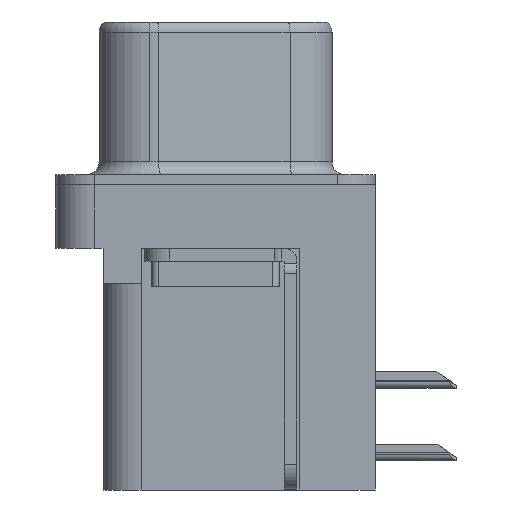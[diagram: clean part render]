
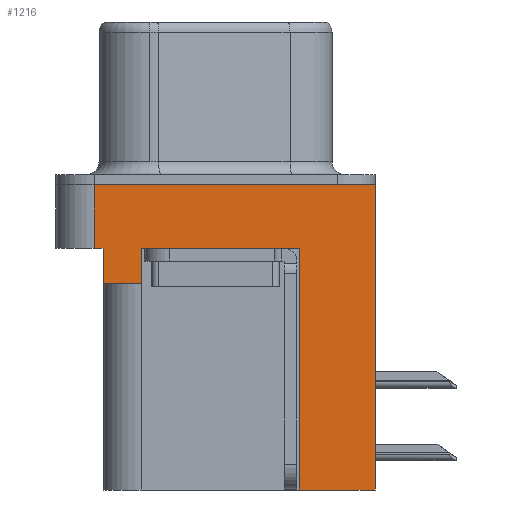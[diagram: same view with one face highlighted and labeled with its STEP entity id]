
A CAD part, left-side view. The second image highlights one B-rep face of the part: STEP entity #1216.
In plain terms, the highlighted planar face has unit normal (-1, 0, 0).
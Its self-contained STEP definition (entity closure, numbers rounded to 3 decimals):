
#251 = DIRECTION ( 'NONE',  ( 0., 0., 1. ) ) ;
#421 = EDGE_CURVE ( 'NONE', #2257, #21516, #5055, .T. ) ;
#840 = VECTOR ( 'NONE', #251, 1000. ) ;
#1216 = ADVANCED_FACE ( 'NONE', ( #18706 ), #11999, .T. ) ;
#1802 = DIRECTION ( 'NONE',  ( 0., 0., 1. ) ) ;
#2257 = VERTEX_POINT ( 'NONE', #19179 ) ;
#2380 = VERTEX_POINT ( 'NONE', #13673 ) ;
#2423 = EDGE_CURVE ( 'NONE', #16780, #21516, #10642, .T. ) ;
#2536 = CARTESIAN_POINT ( 'NONE',  ( -2.91, -6.275, 0. ) ) ;
#3403 = VERTEX_POINT ( 'NONE', #19864 ) ;
#3629 = VERTEX_POINT ( 'NONE', #9405 ) ;
#3684 = LINE ( 'NONE', #2536, #14914 ) ;
#3899 = VECTOR ( 'NONE', #12771, 1000. ) ;
#4153 = CARTESIAN_POINT ( 'NONE',  ( -2.91, 2.895, -3.9 ) ) ;
#4508 = VECTOR ( 'NONE', #14130, 1000. ) ;
#4547 = LINE ( 'NONE', #10882, #23035 ) ;
#4643 = AXIS2_PLACEMENT_3D ( 'NONE', #20243, #8157, #12079 ) ;
#5055 = LINE ( 'NONE', #24226, #22276 ) ;
#5524 = ORIENTED_EDGE ( 'NONE', *, *, #19649, .F. ) ;
#5547 = EDGE_CURVE ( 'NONE', #2380, #3403, #16661, .T. ) ;
#5751 = LINE ( 'NONE', #8375, #22029 ) ;
#6090 = LINE ( 'NONE', #26316, #4508 ) ;
#6662 = EDGE_CURVE ( 'NONE', #9541, #9669, #12764, .T. ) ;
#8157 = DIRECTION ( 'NONE',  ( -1., 0., 0. ) ) ;
#8258 = CARTESIAN_POINT ( 'NONE',  ( -2.91, 4.425, -3.9 ) ) ;
#8375 = CARTESIAN_POINT ( 'NONE',  ( -2.91, -3.295, -12. ) ) ;
#9310 = ORIENTED_EDGE ( 'NONE', *, *, #20270, .F. ) ;
#9405 = CARTESIAN_POINT ( 'NONE',  ( -2.91, 4.775, 0. ) ) ;
#9541 = VERTEX_POINT ( 'NONE', #11743 ) ;
#9669 = VERTEX_POINT ( 'NONE', #13704 ) ;
#9753 = DIRECTION ( 'NONE',  ( 0., 1., 0. ) ) ;
#10254 = LINE ( 'NONE', #24213, #19192 ) ;
#10642 = LINE ( 'NONE', #25937, #10959 ) ;
#10882 = CARTESIAN_POINT ( 'NONE',  ( -2.91, 4.775, -2.5 ) ) ;
#10896 = ORIENTED_EDGE ( 'NONE', *, *, #2423, .T. ) ;
#10959 = VECTOR ( 'NONE', #19844, 1000. ) ;
#11530 = CARTESIAN_POINT ( 'NONE',  ( -2.91, -6.275, -2.5 ) ) ;
#11743 = CARTESIAN_POINT ( 'NONE',  ( -2.91, 4.775, -2.5 ) ) ;
#11999 = PLANE ( 'NONE',  #4643 ) ;
#12079 = DIRECTION ( 'NONE',  ( 0., 0., 1. ) ) ;
#12124 = CARTESIAN_POINT ( 'NONE',  ( -2.91, 4.425, -3.9 ) ) ;
#12764 = LINE ( 'NONE', #11530, #18198 ) ;
#12771 = DIRECTION ( 'NONE',  ( 0., 0., 1. ) ) ;
#13673 = CARTESIAN_POINT ( 'NONE',  ( -2.91, -6.275, -12. ) ) ;
#13704 = CARTESIAN_POINT ( 'NONE',  ( -2.91, 4.425, -2.5 ) ) ;
#14130 = DIRECTION ( 'NONE',  ( 0., 0., 1. ) ) ;
#14210 = CARTESIAN_POINT ( 'NONE',  ( -2.91, -3.295, -2.5 ) ) ;
#14914 = VECTOR ( 'NONE', #24719, 1000. ) ;
#16099 = ORIENTED_EDGE ( 'NONE', *, *, #18065, .F. ) ;
#16661 = LINE ( 'NONE', #26484, #3899 ) ;
#16780 = VERTEX_POINT ( 'NONE', #18394 ) ;
#18065 = EDGE_CURVE ( 'NONE', #23569, #22270, #10254, .T. ) ;
#18198 = VECTOR ( 'NONE', #23469, 1000. ) ;
#18248 = EDGE_CURVE ( 'NONE', #2380, #2257, #5751, .T. ) ;
#18394 = CARTESIAN_POINT ( 'NONE',  ( -2.91, 2.895, -2.5 ) ) ;
#18706 = FACE_OUTER_BOUND ( 'NONE', #19726, .T. ) ;
#19179 = CARTESIAN_POINT ( 'NONE',  ( -2.91, -3.295, -12. ) ) ;
#19192 = VECTOR ( 'NONE', #9753, 1000. ) ;
#19393 = ORIENTED_EDGE ( 'NONE', *, *, #25135, .T. ) ;
#19649 = EDGE_CURVE ( 'NONE', #22270, #9669, #25145, .T. ) ;
#19726 = EDGE_LOOP ( 'NONE', ( #9310, #20275, #21149, #5524, #16099, #19393, #10896, #19888, #24588, #23963 ) ) ;
#19844 = DIRECTION ( 'NONE',  ( 0., -1., 0. ) ) ;
#19864 = CARTESIAN_POINT ( 'NONE',  ( -2.91, -6.275, 0. ) ) ;
#19888 = ORIENTED_EDGE ( 'NONE', *, *, #421, .F. ) ;
#20243 = CARTESIAN_POINT ( 'NONE',  ( -2.91, -6.275, -2.5 ) ) ;
#20270 = EDGE_CURVE ( 'NONE', #3629, #3403, #3684, .T. ) ;
#20275 = ORIENTED_EDGE ( 'NONE', *, *, #21636, .F. ) ;
#20986 = DIRECTION ( 'NONE',  ( 0., 1., 0. ) ) ;
#21095 = DIRECTION ( 'NONE',  ( 0., 0., 1. ) ) ;
#21149 = ORIENTED_EDGE ( 'NONE', *, *, #6662, .T. ) ;
#21516 = VERTEX_POINT ( 'NONE', #14210 ) ;
#21636 = EDGE_CURVE ( 'NONE', #9541, #3629, #4547, .T. ) ;
#22029 = VECTOR ( 'NONE', #20986, 1000. ) ;
#22270 = VERTEX_POINT ( 'NONE', #8258 ) ;
#22276 = VECTOR ( 'NONE', #1802, 1000. ) ;
#23035 = VECTOR ( 'NONE', #21095, 1000. ) ;
#23469 = DIRECTION ( 'NONE',  ( 0., -1., 0. ) ) ;
#23569 = VERTEX_POINT ( 'NONE', #4153 ) ;
#23963 = ORIENTED_EDGE ( 'NONE', *, *, #5547, .T. ) ;
#24213 = CARTESIAN_POINT ( 'NONE',  ( -2.91, 4.425, -3.9 ) ) ;
#24226 = CARTESIAN_POINT ( 'NONE',  ( -2.91, -3.295, -12. ) ) ;
#24588 = ORIENTED_EDGE ( 'NONE', *, *, #18248, .F. ) ;
#24719 = DIRECTION ( 'NONE',  ( 0., -1., 0. ) ) ;
#25135 = EDGE_CURVE ( 'NONE', #23569, #16780, #6090, .T. ) ;
#25145 = LINE ( 'NONE', #12124, #840 ) ;
#25937 = CARTESIAN_POINT ( 'NONE',  ( -2.91, -6.275, -2.5 ) ) ;
#26316 = CARTESIAN_POINT ( 'NONE',  ( -2.91, 2.895, -3.9 ) ) ;
#26484 = CARTESIAN_POINT ( 'NONE',  ( -2.91, -6.275, -2.5 ) ) ;
